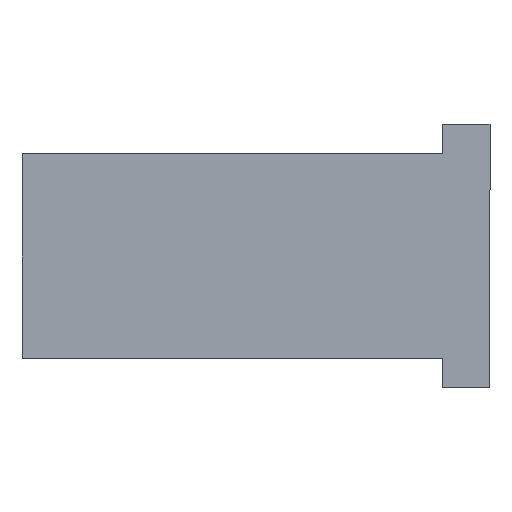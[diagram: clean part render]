
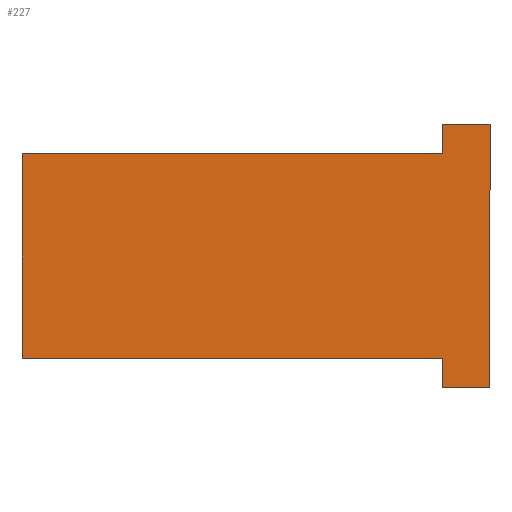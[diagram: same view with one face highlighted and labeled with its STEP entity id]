
A CAD part, front view. The second image highlights one B-rep face of the part: STEP entity #227.
In plain terms, the highlighted planar face has unit normal (0, -1, 0).
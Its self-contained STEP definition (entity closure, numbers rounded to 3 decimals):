
#24 = CARTESIAN_POINT ( 'NONE',  ( 21.64, 0., 6.085 ) ) ;
#28 = DIRECTION ( 'NONE',  ( -1., 0., 0. ) ) ;
#29 = ORIENTED_EDGE ( 'NONE', *, *, #135, .F. ) ;
#39 = CARTESIAN_POINT ( 'NONE',  ( 0., 0., -4.725 ) ) ;
#41 = EDGE_CURVE ( 'NONE', #230, #312, #213, .T. ) ;
#42 = EDGE_CURVE ( 'NONE', #131, #230, #268, .T. ) ;
#50 = EDGE_CURVE ( 'NONE', #283, #238, #320, .T. ) ;
#53 = DIRECTION ( 'NONE',  ( 0., 0., 1. ) ) ;
#58 = EDGE_LOOP ( 'NONE', ( #183, #148, #184, #134, #262, #130, #29, #128 ) ) ;
#59 = LINE ( 'NONE', #110, #91 ) ;
#62 = VECTOR ( 'NONE', #137, 1000. ) ;
#70 = CARTESIAN_POINT ( 'NONE',  ( 19.46, 0., -4.725 ) ) ;
#73 = CARTESIAN_POINT ( 'NONE',  ( 0., 0., 4.725 ) ) ;
#91 = VECTOR ( 'NONE', #180, 1000. ) ;
#92 = DIRECTION ( 'NONE',  ( 0., 0., -1. ) ) ;
#96 = PLANE ( 'NONE',  #247 ) ;
#100 = EDGE_CURVE ( 'NONE', #238, #131, #129, .T. ) ;
#101 = CARTESIAN_POINT ( 'NONE',  ( 19.46, 0., 6.085 ) ) ;
#110 = CARTESIAN_POINT ( 'NONE',  ( 21.64, 0., -6.085 ) ) ;
#111 = CARTESIAN_POINT ( 'NONE',  ( 21.64, 0., -6.085 ) ) ;
#128 = ORIENTED_EDGE ( 'NONE', *, *, #185, .F. ) ;
#129 = LINE ( 'NONE', #332, #271 ) ;
#130 = ORIENTED_EDGE ( 'NONE', *, *, #280, .F. ) ;
#131 = VERTEX_POINT ( 'NONE', #254 ) ;
#133 = CARTESIAN_POINT ( 'NONE',  ( 0., 0., 4.725 ) ) ;
#134 = ORIENTED_EDGE ( 'NONE', *, *, #50, .F. ) ;
#135 = EDGE_CURVE ( 'NONE', #152, #178, #202, .T. ) ;
#137 = DIRECTION ( 'NONE',  ( 0., 0., 1. ) ) ;
#139 = CARTESIAN_POINT ( 'NONE',  ( 0., 0., 0. ) ) ;
#145 = DIRECTION ( 'NONE',  ( 0., 0., 1. ) ) ;
#148 = ORIENTED_EDGE ( 'NONE', *, *, #42, .F. ) ;
#152 = VERTEX_POINT ( 'NONE', #101 ) ;
#159 = VECTOR ( 'NONE', #310, 1000. ) ;
#162 = VERTEX_POINT ( 'NONE', #111 ) ;
#167 = FACE_OUTER_BOUND ( 'NONE', #58, .T. ) ;
#168 = LINE ( 'NONE', #193, #296 ) ;
#169 = VECTOR ( 'NONE', #237, 1000. ) ;
#178 = VERTEX_POINT ( 'NONE', #24 ) ;
#180 = DIRECTION ( 'NONE',  ( -1., 0., 0. ) ) ;
#183 = ORIENTED_EDGE ( 'NONE', *, *, #41, .F. ) ;
#184 = ORIENTED_EDGE ( 'NONE', *, *, #100, .F. ) ;
#185 = EDGE_CURVE ( 'NONE', #312, #152, #218, .T. ) ;
#193 = CARTESIAN_POINT ( 'NONE',  ( 21.64, 0., 6.085 ) ) ;
#195 = DIRECTION ( 'NONE',  ( 0., -1., 0. ) ) ;
#197 = DIRECTION ( 'NONE',  ( 0., 0., -1. ) ) ;
#202 = LINE ( 'NONE', #334, #159 ) ;
#213 = LINE ( 'NONE', #133, #169 ) ;
#214 = VECTOR ( 'NONE', #53, 1000. ) ;
#218 = LINE ( 'NONE', #306, #309 ) ;
#227 = ADVANCED_FACE ( 'NONE', ( #167 ), #96, .T. ) ;
#228 = CARTESIAN_POINT ( 'NONE',  ( 19.46, 0., 4.725 ) ) ;
#230 = VERTEX_POINT ( 'NONE', #73 ) ;
#237 = DIRECTION ( 'NONE',  ( 1., 0., 0. ) ) ;
#238 = VERTEX_POINT ( 'NONE', #70 ) ;
#247 = AXIS2_PLACEMENT_3D ( 'NONE', #139, #195, #197 ) ;
#254 = CARTESIAN_POINT ( 'NONE',  ( 0., 0., -4.725 ) ) ;
#262 = ORIENTED_EDGE ( 'NONE', *, *, #319, .F. ) ;
#268 = LINE ( 'NONE', #39, #62 ) ;
#271 = VECTOR ( 'NONE', #28, 1000. ) ;
#276 = CARTESIAN_POINT ( 'NONE',  ( 19.46, 0., -6.085 ) ) ;
#280 = EDGE_CURVE ( 'NONE', #178, #162, #168, .T. ) ;
#283 = VERTEX_POINT ( 'NONE', #276 ) ;
#284 = CARTESIAN_POINT ( 'NONE',  ( 19.46, 0., -6.085 ) ) ;
#296 = VECTOR ( 'NONE', #92, 1000. ) ;
#306 = CARTESIAN_POINT ( 'NONE',  ( 19.46, 0., 4.725 ) ) ;
#309 = VECTOR ( 'NONE', #145, 1000. ) ;
#310 = DIRECTION ( 'NONE',  ( 1., 0., 0. ) ) ;
#312 = VERTEX_POINT ( 'NONE', #228 ) ;
#319 = EDGE_CURVE ( 'NONE', #162, #283, #59, .T. ) ;
#320 = LINE ( 'NONE', #284, #214 ) ;
#332 = CARTESIAN_POINT ( 'NONE',  ( 19.46, 0., -4.725 ) ) ;
#334 = CARTESIAN_POINT ( 'NONE',  ( 19.46, 0., 6.085 ) ) ;
